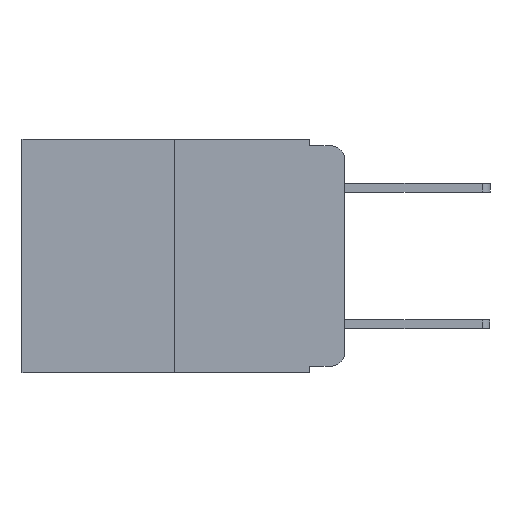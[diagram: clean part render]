
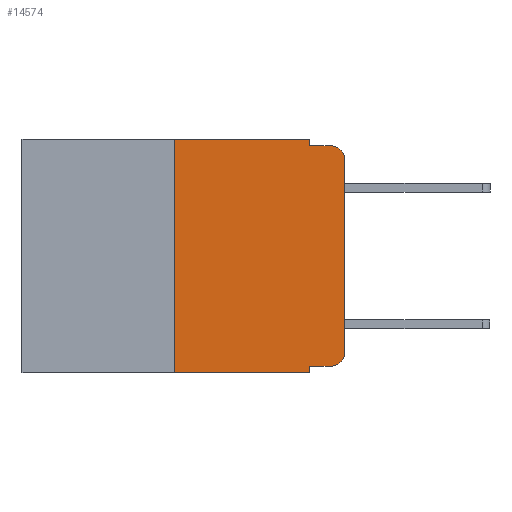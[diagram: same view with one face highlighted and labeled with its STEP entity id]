
A CAD part, left-side view. The second image highlights one B-rep face of the part: STEP entity #14574.
In plain terms, the highlighted planar face has unit normal (-1, 0, 0).
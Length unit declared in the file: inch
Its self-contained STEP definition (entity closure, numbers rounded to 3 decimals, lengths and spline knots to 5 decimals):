
#165 = EDGE_CURVE ( 'NONE', #5831, #4792, #11622, .T. ) ;
#669 = VERTEX_POINT ( 'NONE', #8501 ) ;
#972 = PLANE ( 'NONE',  #5659 ) ;
#1027 = AXIS2_PLACEMENT_3D ( 'NONE', #14235, #4806, #15732 ) ;
#1198 = LINE ( 'NONE', #18903, #12711 ) ;
#1745 = DIRECTION ( 'NONE',  ( 0., -1., 0. ) ) ;
#2481 = VECTOR ( 'NONE', #1745, 39.37008 ) ;
#3145 = VERTEX_POINT ( 'NONE', #7598 ) ;
#3214 = CARTESIAN_POINT ( 'NONE',  ( 0., 0., -0.313 ) ) ;
#3637 = VECTOR ( 'NONE', #9012, 39.37008 ) ;
#4226 = CARTESIAN_POINT ( 'NONE',  ( 0., 0.051, -0.333 ) ) ;
#4401 = DIRECTION ( 'NONE',  ( 0., -1., 0. ) ) ;
#4538 = CARTESIAN_POINT ( 'NONE',  ( 0., 0.473, 0. ) ) ;
#4620 = VECTOR ( 'NONE', #9293, 39.37008 ) ;
#4710 = ORIENTED_EDGE ( 'NONE', *, *, #14147, .F. ) ;
#4751 = LINE ( 'NONE', #7424, #3637 ) ;
#4792 = VERTEX_POINT ( 'NONE', #20214 ) ;
#4806 = DIRECTION ( 'NONE',  ( -1., 0., 0. ) ) ;
#4837 = CARTESIAN_POINT ( 'NONE',  ( 0., 0.473, 0. ) ) ;
#5092 = VERTEX_POINT ( 'NONE', #4226 ) ;
#5163 = LINE ( 'NONE', #12361, #4620 ) ;
#5219 = EDGE_CURVE ( 'NONE', #9406, #14464, #13444, .T. ) ;
#5245 = VERTEX_POINT ( 'NONE', #3214 ) ;
#5332 = DIRECTION ( 'NONE',  ( -1., 0., 0. ) ) ;
#5449 = CARTESIAN_POINT ( 'NONE',  ( 0., 0.473, -0.343 ) ) ;
#5659 = AXIS2_PLACEMENT_3D ( 'NONE', #4538, #15501, #6232 ) ;
#5831 = VERTEX_POINT ( 'NONE', #15018 ) ;
#5872 = CARTESIAN_POINT ( 'NONE',  ( 0., 0.051, 0. ) ) ;
#5892 = EDGE_LOOP ( 'NONE', ( #14310, #6524, #20479, #4710, #8963, #9464, #17556, #14086, #6286, #7750 ) ) ;
#6101 = CARTESIAN_POINT ( 'NONE',  ( 0., 0.051, -0.333 ) ) ;
#6232 = DIRECTION ( 'NONE',  ( 0., 0., -1. ) ) ;
#6286 = ORIENTED_EDGE ( 'NONE', *, *, #11022, .T. ) ;
#6397 = VECTOR ( 'NONE', #19437, 39.37008 ) ;
#6524 = ORIENTED_EDGE ( 'NONE', *, *, #17144, .T. ) ;
#7312 = CARTESIAN_POINT ( 'NONE',  ( 0., 0.25, 0. ) ) ;
#7424 = CARTESIAN_POINT ( 'NONE',  ( 0., 0.051, -0.01 ) ) ;
#7582 = VECTOR ( 'NONE', #16425, 39.37008 ) ;
#7598 = CARTESIAN_POINT ( 'NONE',  ( 0., 0.02, -0.01 ) ) ;
#7750 = ORIENTED_EDGE ( 'NONE', *, *, #9989, .T. ) ;
#8501 = CARTESIAN_POINT ( 'NONE',  ( 0., 0., -0.03 ) ) ;
#8690 = CARTESIAN_POINT ( 'NONE',  ( 0., 0.051, -0.01 ) ) ;
#8963 = ORIENTED_EDGE ( 'NONE', *, *, #5219, .F. ) ;
#8989 = AXIS2_PLACEMENT_3D ( 'NONE', #14704, #5332, #16177 ) ;
#9012 = DIRECTION ( 'NONE',  ( 0., -1., 0. ) ) ;
#9293 = DIRECTION ( 'NONE',  ( 0., 0., -1. ) ) ;
#9406 = VERTEX_POINT ( 'NONE', #9646 ) ;
#9464 = ORIENTED_EDGE ( 'NONE', *, *, #13117, .F. ) ;
#9525 = FACE_OUTER_BOUND ( 'NONE', #5892, .T. ) ;
#9646 = CARTESIAN_POINT ( 'NONE',  ( 0., 0.25, 0. ) ) ;
#9655 = DIRECTION ( 'NONE',  ( 0., -1., 0. ) ) ;
#9989 = EDGE_CURVE ( 'NONE', #15224, #5245, #18905, .T. ) ;
#10651 = LINE ( 'NONE', #6101, #18186 ) ;
#11022 = EDGE_CURVE ( 'NONE', #5092, #15224, #10651, .T. ) ;
#11622 = LINE ( 'NONE', #5449, #2481 ) ;
#12079 = EDGE_CURVE ( 'NONE', #5092, #4792, #5163, .T. ) ;
#12361 = CARTESIAN_POINT ( 'NONE',  ( 0., 0.051, 0. ) ) ;
#12472 = VECTOR ( 'NONE', #9655, 39.37008 ) ;
#12711 = VECTOR ( 'NONE', #20341, 39.37008 ) ;
#13117 = EDGE_CURVE ( 'NONE', #5831, #9406, #14667, .T. ) ;
#13444 = LINE ( 'NONE', #4837, #12472 ) ;
#14086 = ORIENTED_EDGE ( 'NONE', *, *, #12079, .F. ) ;
#14147 = EDGE_CURVE ( 'NONE', #14464, #18912, #1198, .T. ) ;
#14235 = CARTESIAN_POINT ( 'NONE',  ( 0., 0.02, -0.313 ) ) ;
#14310 = ORIENTED_EDGE ( 'NONE', *, *, #18083, .T. ) ;
#14442 = CIRCLE ( 'NONE', #8989, 0.02 ) ;
#14464 = VERTEX_POINT ( 'NONE', #5872 ) ;
#14574 = ADVANCED_FACE ( 'NONE', ( #9525 ), #972, .F. ) ;
#14667 = LINE ( 'NONE', #7312, #6397 ) ;
#14704 = CARTESIAN_POINT ( 'NONE',  ( 0., 0.02, -0.03 ) ) ;
#14938 = CARTESIAN_POINT ( 'NONE',  ( 0., 0., 0. ) ) ;
#15018 = CARTESIAN_POINT ( 'NONE',  ( 0., 0.25, -0.343 ) ) ;
#15141 = EDGE_CURVE ( 'NONE', #18912, #3145, #4751, .T. ) ;
#15224 = VERTEX_POINT ( 'NONE', #15339 ) ;
#15339 = CARTESIAN_POINT ( 'NONE',  ( 0., 0.02, -0.333 ) ) ;
#15501 = DIRECTION ( 'NONE',  ( 1., 0., 0. ) ) ;
#15732 = DIRECTION ( 'NONE',  ( 0., 0., -1. ) ) ;
#15801 = LINE ( 'NONE', #14938, #7582 ) ;
#16177 = DIRECTION ( 'NONE',  ( 0., 0., -1. ) ) ;
#16425 = DIRECTION ( 'NONE',  ( 0., 0., 1. ) ) ;
#17144 = EDGE_CURVE ( 'NONE', #669, #3145, #14442, .T. ) ;
#17556 = ORIENTED_EDGE ( 'NONE', *, *, #165, .T. ) ;
#18083 = EDGE_CURVE ( 'NONE', #5245, #669, #15801, .T. ) ;
#18186 = VECTOR ( 'NONE', #4401, 39.37008 ) ;
#18903 = CARTESIAN_POINT ( 'NONE',  ( 0., 0.051, 0. ) ) ;
#18905 = CIRCLE ( 'NONE', #1027, 0.02 ) ;
#18912 = VERTEX_POINT ( 'NONE', #8690 ) ;
#19437 = DIRECTION ( 'NONE',  ( 0., 0., 1. ) ) ;
#20214 = CARTESIAN_POINT ( 'NONE',  ( 0., 0.051, -0.343 ) ) ;
#20341 = DIRECTION ( 'NONE',  ( 0., 0., -1. ) ) ;
#20479 = ORIENTED_EDGE ( 'NONE', *, *, #15141, .F. ) ;
